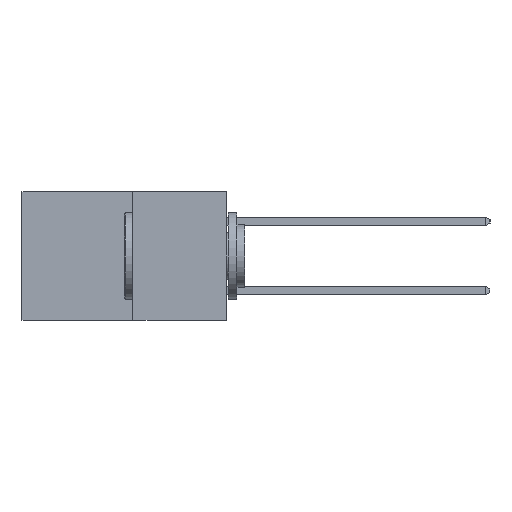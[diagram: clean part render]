
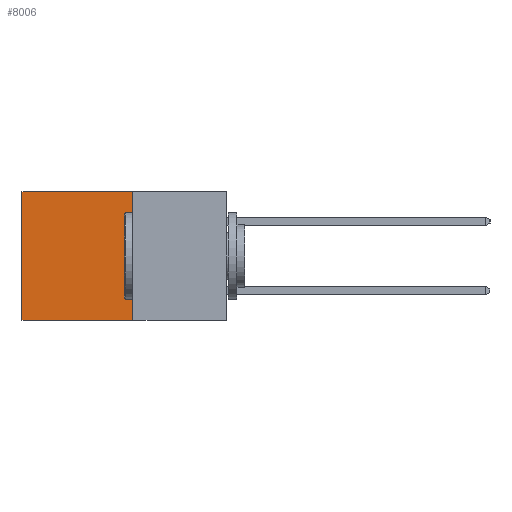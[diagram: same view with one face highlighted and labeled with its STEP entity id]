
A CAD part, left-side view. The second image highlights one B-rep face of the part: STEP entity #8006.
In plain terms, the highlighted planar face has unit normal (-1, 0, 0).
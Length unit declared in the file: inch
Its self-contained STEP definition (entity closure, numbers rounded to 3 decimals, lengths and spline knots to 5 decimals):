
#87 = ORIENTED_EDGE ( 'NONE', *, *, #9792, .T. ) ;
#224 = DIRECTION ( 'NONE',  ( 0., 0., -1. ) ) ;
#505 = ORIENTED_EDGE ( 'NONE', *, *, #6135, .F. ) ;
#514 = FACE_OUTER_BOUND ( 'NONE', #740, .T. ) ;
#740 = EDGE_LOOP ( 'NONE', ( #87, #3218, #505, #3059 ) ) ;
#1063 = LINE ( 'NONE', #7643, #2921 ) ;
#1579 = LINE ( 'NONE', #9006, #10710 ) ;
#1951 = AXIS2_PLACEMENT_3D ( 'NONE', #1956, #4659, #10801 ) ;
#1956 = CARTESIAN_POINT ( 'NONE',  ( 0.277, 0.27, -0.37 ) ) ;
#2243 = VECTOR ( 'NONE', #224, 39.37008 ) ;
#2533 = LINE ( 'NONE', #10993, #2243 ) ;
#2827 = DIRECTION ( 'NONE',  ( 0., 0., -1. ) ) ;
#2921 = VECTOR ( 'NONE', #10313, 39.37008 ) ;
#2944 = CARTESIAN_POINT ( 'NONE',  ( 0.277, 0.59, -0.37 ) ) ;
#3059 = ORIENTED_EDGE ( 'NONE', *, *, #6257, .T. ) ;
#3218 = ORIENTED_EDGE ( 'NONE', *, *, #4285, .F. ) ;
#3523 = VERTEX_POINT ( 'NONE', #4889 ) ;
#4081 = LINE ( 'NONE', #9328, #10577 ) ;
#4285 = EDGE_CURVE ( 'NONE', #10524, #7439, #4081, .T. ) ;
#4659 = DIRECTION ( 'NONE',  ( 1., 0., 0. ) ) ;
#4846 = VERTEX_POINT ( 'NONE', #6311 ) ;
#4889 = CARTESIAN_POINT ( 'NONE',  ( 0.277, 0.59, 0. ) ) ;
#6135 = EDGE_CURVE ( 'NONE', #4846, #10524, #2533, .T. ) ;
#6217 = CARTESIAN_POINT ( 'NONE',  ( 0.277, 0.27, -0.37 ) ) ;
#6257 = EDGE_CURVE ( 'NONE', #4846, #3523, #1063, .T. ) ;
#6311 = CARTESIAN_POINT ( 'NONE',  ( 0.277, 0.27, 0. ) ) ;
#7439 = VERTEX_POINT ( 'NONE', #2944 ) ;
#7643 = CARTESIAN_POINT ( 'NONE',  ( 0.277, 0.27, 0. ) ) ;
#8006 = ADVANCED_FACE ( 'NONE', ( #514 ), #9918, .F. ) ;
#9006 = CARTESIAN_POINT ( 'NONE',  ( 0.277, 0.59, -0.37 ) ) ;
#9298 = DIRECTION ( 'NONE',  ( 0., 1., 0. ) ) ;
#9328 = CARTESIAN_POINT ( 'NONE',  ( 0.277, 0.27, -0.37 ) ) ;
#9792 = EDGE_CURVE ( 'NONE', #3523, #7439, #1579, .T. ) ;
#9918 = PLANE ( 'NONE',  #1951 ) ;
#10313 = DIRECTION ( 'NONE',  ( 0., 1., 0. ) ) ;
#10524 = VERTEX_POINT ( 'NONE', #6217 ) ;
#10577 = VECTOR ( 'NONE', #9298, 39.37008 ) ;
#10710 = VECTOR ( 'NONE', #2827, 39.37008 ) ;
#10801 = DIRECTION ( 'NONE',  ( 0., 0., -1. ) ) ;
#10993 = CARTESIAN_POINT ( 'NONE',  ( 0.277, 0.27, -0.37 ) ) ;
